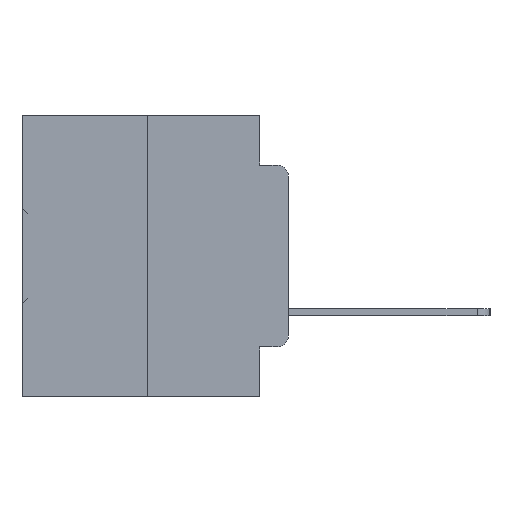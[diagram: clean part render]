
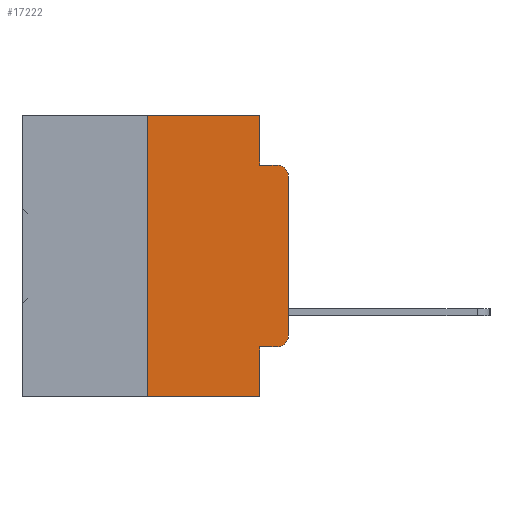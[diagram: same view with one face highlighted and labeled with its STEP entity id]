
A CAD part, left-side view. The second image highlights one B-rep face of the part: STEP entity #17222.
In plain terms, the highlighted planar face has unit normal (-1, 0, 0).
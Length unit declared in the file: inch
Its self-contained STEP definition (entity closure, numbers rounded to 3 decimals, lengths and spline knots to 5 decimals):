
#42 = LINE ( 'NONE', #22701, #21802 ) ;
#68 = CARTESIAN_POINT ( 'NONE',  ( 0., 0.051, -0.4115 ) ) ;
#921 = ORIENTED_EDGE ( 'NONE', *, *, #29462, .T. ) ;
#1010 = ORIENTED_EDGE ( 'NONE', *, *, #8802, .T. ) ;
#1941 = DIRECTION ( 'NONE',  ( 0., -1., 0. ) ) ;
#2114 = CARTESIAN_POINT ( 'NONE',  ( 0., 0.473, 0. ) ) ;
#3270 = CARTESIAN_POINT ( 'NONE',  ( 0., 0., 0. ) ) ;
#3624 = DIRECTION ( 'NONE',  ( 0., 0., 1. ) ) ;
#3947 = LINE ( 'NONE', #3270, #9522 ) ;
#4483 = EDGE_CURVE ( 'NONE', #27647, #27212, #23643, .T. ) ;
#4816 = CARTESIAN_POINT ( 'NONE',  ( 0., 0.02, -0.4115 ) ) ;
#4856 = DIRECTION ( 'NONE',  ( 0., -1., 0. ) ) ;
#5163 = CARTESIAN_POINT ( 'NONE',  ( 0., 0.051, 0. ) ) ;
#5337 = CIRCLE ( 'NONE', #15021, 0.02 ) ;
#5418 = ORIENTED_EDGE ( 'NONE', *, *, #26571, .F. ) ;
#5436 = CARTESIAN_POINT ( 'NONE',  ( 0., 0.02, -0.0885 ) ) ;
#5619 = DIRECTION ( 'NONE',  ( 0., -1., 0. ) ) ;
#5774 = ORIENTED_EDGE ( 'NONE', *, *, #10663, .F. ) ;
#5942 = VERTEX_POINT ( 'NONE', #16817 ) ;
#7921 = DIRECTION ( 'NONE',  ( 0., 0., -1. ) ) ;
#7965 = CARTESIAN_POINT ( 'NONE',  ( 0., 0.051, -0.0885 ) ) ;
#7982 = VERTEX_POINT ( 'NONE', #12613 ) ;
#8802 = EDGE_CURVE ( 'NONE', #20246, #33603, #3947, .T. ) ;
#9039 = EDGE_CURVE ( 'NONE', #27647, #12112, #10783, .T. ) ;
#9522 = VECTOR ( 'NONE', #14024, 39.37008 ) ;
#9844 = VECTOR ( 'NONE', #7921, 39.37008 ) ;
#10634 = LINE ( 'NONE', #2114, #15337 ) ;
#10663 = EDGE_CURVE ( 'NONE', #7982, #16407, #42, .T. ) ;
#10783 = LINE ( 'NONE', #12228, #31498 ) ;
#10951 = DIRECTION ( 'NONE',  ( -1., 0., 0. ) ) ;
#10959 = DIRECTION ( 'NONE',  ( 0., -1., 0. ) ) ;
#11019 = EDGE_CURVE ( 'NONE', #5942, #11674, #31406, .T. ) ;
#11674 = VERTEX_POINT ( 'NONE', #7965 ) ;
#12112 = VERTEX_POINT ( 'NONE', #33818 ) ;
#12163 = ORIENTED_EDGE ( 'NONE', *, *, #34093, .T. ) ;
#12228 = CARTESIAN_POINT ( 'NONE',  ( 0., 0.051, 0. ) ) ;
#12613 = CARTESIAN_POINT ( 'NONE',  ( 0., 0.25, -0.5 ) ) ;
#13354 = DIRECTION ( 'NONE',  ( 0., 0., -1. ) ) ;
#13855 = CARTESIAN_POINT ( 'NONE',  ( 0., 0.473, -0.5 ) ) ;
#14024 = DIRECTION ( 'NONE',  ( 0., 0., 1. ) ) ;
#14355 = CARTESIAN_POINT ( 'NONE',  ( 0., 0.02, -0.3915 ) ) ;
#14558 = VERTEX_POINT ( 'NONE', #5436 ) ;
#15021 = AXIS2_PLACEMENT_3D ( 'NONE', #27231, #10951, #29901 ) ;
#15337 = VECTOR ( 'NONE', #4856, 39.37008 ) ;
#15621 = AXIS2_PLACEMENT_3D ( 'NONE', #14355, #33142, #17113 ) ;
#16407 = VERTEX_POINT ( 'NONE', #24236 ) ;
#16415 = LINE ( 'NONE', #21021, #18097 ) ;
#16451 = VECTOR ( 'NONE', #10959, 39.37008 ) ;
#16817 = CARTESIAN_POINT ( 'NONE',  ( 0., 0.051, 0. ) ) ;
#17113 = DIRECTION ( 'NONE',  ( 0., 0., -1. ) ) ;
#17222 = ADVANCED_FACE ( 'NONE', ( #31517 ), #24163, .F. ) ;
#17281 = AXIS2_PLACEMENT_3D ( 'NONE', #26864, #29558, #13354 ) ;
#17737 = ORIENTED_EDGE ( 'NONE', *, *, #28915, .T. ) ;
#18097 = VECTOR ( 'NONE', #1941, 39.37008 ) ;
#18304 = ORIENTED_EDGE ( 'NONE', *, *, #32968, .F. ) ;
#18627 = LINE ( 'NONE', #13855, #32058 ) ;
#20246 = VERTEX_POINT ( 'NONE', #30912 ) ;
#20658 = EDGE_LOOP ( 'NONE', ( #1010, #921, #18304, #30087, #5418, #5774, #17737, #27035, #34023, #12163 ) ) ;
#21021 = CARTESIAN_POINT ( 'NONE',  ( 0., 0.051, -0.0885 ) ) ;
#21390 = CIRCLE ( 'NONE', #15621, 0.02 ) ;
#21802 = VECTOR ( 'NONE', #3624, 39.37008 ) ;
#22701 = CARTESIAN_POINT ( 'NONE',  ( 0., 0.25, 0. ) ) ;
#23643 = LINE ( 'NONE', #68, #16451 ) ;
#24163 = PLANE ( 'NONE',  #17281 ) ;
#24236 = CARTESIAN_POINT ( 'NONE',  ( 0., 0.25, 0. ) ) ;
#26571 = EDGE_CURVE ( 'NONE', #16407, #5942, #10634, .T. ) ;
#26864 = CARTESIAN_POINT ( 'NONE',  ( 0., 0.473, 0. ) ) ;
#27035 = ORIENTED_EDGE ( 'NONE', *, *, #9039, .F. ) ;
#27212 = VERTEX_POINT ( 'NONE', #4816 ) ;
#27231 = CARTESIAN_POINT ( 'NONE',  ( 0., 0.02, -0.1085 ) ) ;
#27647 = VERTEX_POINT ( 'NONE', #28557 ) ;
#28557 = CARTESIAN_POINT ( 'NONE',  ( 0., 0.051, -0.4115 ) ) ;
#28572 = DIRECTION ( 'NONE',  ( 0., 0., -1. ) ) ;
#28915 = EDGE_CURVE ( 'NONE', #7982, #12112, #18627, .T. ) ;
#29462 = EDGE_CURVE ( 'NONE', #33603, #14558, #5337, .T. ) ;
#29558 = DIRECTION ( 'NONE',  ( 1., 0., 0. ) ) ;
#29589 = CARTESIAN_POINT ( 'NONE',  ( 0., 0., -0.1085 ) ) ;
#29901 = DIRECTION ( 'NONE',  ( 0., 0., -1. ) ) ;
#30087 = ORIENTED_EDGE ( 'NONE', *, *, #11019, .F. ) ;
#30912 = CARTESIAN_POINT ( 'NONE',  ( 0., 0., -0.3915 ) ) ;
#31406 = LINE ( 'NONE', #5163, #9844 ) ;
#31498 = VECTOR ( 'NONE', #28572, 39.37008 ) ;
#31517 = FACE_OUTER_BOUND ( 'NONE', #20658, .T. ) ;
#32058 = VECTOR ( 'NONE', #5619, 39.37008 ) ;
#32968 = EDGE_CURVE ( 'NONE', #11674, #14558, #16415, .T. ) ;
#33142 = DIRECTION ( 'NONE',  ( -1., 0., 0. ) ) ;
#33603 = VERTEX_POINT ( 'NONE', #29589 ) ;
#33818 = CARTESIAN_POINT ( 'NONE',  ( 0., 0.051, -0.5 ) ) ;
#34023 = ORIENTED_EDGE ( 'NONE', *, *, #4483, .T. ) ;
#34093 = EDGE_CURVE ( 'NONE', #27212, #20246, #21390, .T. ) ;
